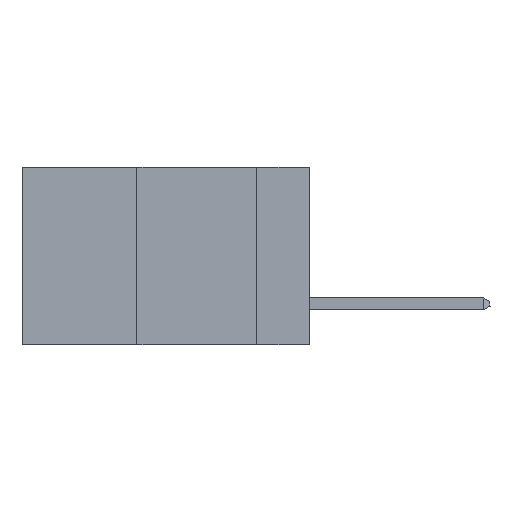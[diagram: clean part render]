
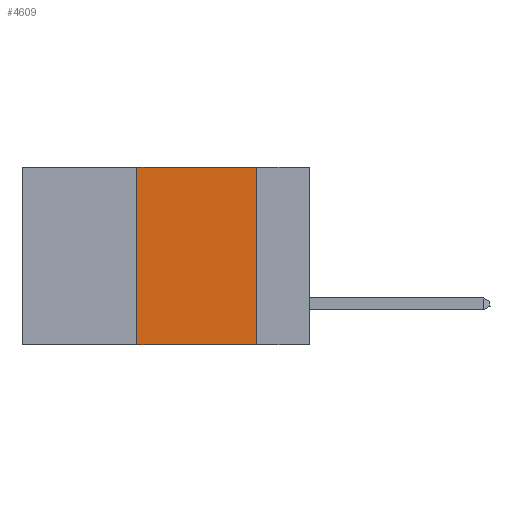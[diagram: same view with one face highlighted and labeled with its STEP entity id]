
A CAD part, left-side view. The second image highlights one B-rep face of the part: STEP entity #4609.
In plain terms, the highlighted planar face has unit normal (-1, 0, 0).
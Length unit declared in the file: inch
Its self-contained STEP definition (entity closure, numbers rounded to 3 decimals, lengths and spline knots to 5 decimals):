
#350 = VECTOR ( 'NONE', #17200, 39.37008 ) ;
#497 = VERTEX_POINT ( 'NONE', #6033 ) ;
#723 = AXIS2_PLACEMENT_3D ( 'NONE', #917, #4396, #20403 ) ;
#917 = CARTESIAN_POINT ( 'NONE',  ( 0., 0.6, 0. ) ) ;
#1806 = EDGE_CURVE ( 'NONE', #2650, #6221, #4624, .T. ) ;
#2217 = EDGE_CURVE ( 'NONE', #2650, #497, #7634, .T. ) ;
#2650 = VERTEX_POINT ( 'NONE', #16991 ) ;
#2866 = ORIENTED_EDGE ( 'NONE', *, *, #17367, .F. ) ;
#3147 = VERTEX_POINT ( 'NONE', #14581 ) ;
#3771 = VECTOR ( 'NONE', #6370, 39.37008 ) ;
#3840 = CARTESIAN_POINT ( 'NONE',  ( 0., 0.11, -0.37 ) ) ;
#4396 = DIRECTION ( 'NONE',  ( 1., 0., 0. ) ) ;
#4609 = ADVANCED_FACE ( 'NONE', ( #16020 ), #13310, .F. ) ;
#4624 = LINE ( 'NONE', #15113, #9568 ) ;
#5716 = EDGE_LOOP ( 'NONE', ( #9611, #2866, #8978, #10010 ) ) ;
#5736 = LINE ( 'NONE', #20801, #6278 ) ;
#6033 = CARTESIAN_POINT ( 'NONE',  ( 0., 0.36, 0. ) ) ;
#6221 = VERTEX_POINT ( 'NONE', #3840 ) ;
#6278 = VECTOR ( 'NONE', #22473, 39.37008 ) ;
#6370 = DIRECTION ( 'NONE',  ( 0., 0., 1. ) ) ;
#7634 = LINE ( 'NONE', #20424, #3771 ) ;
#8950 = LINE ( 'NONE', #22598, #350 ) ;
#8978 = ORIENTED_EDGE ( 'NONE', *, *, #2217, .F. ) ;
#9568 = VECTOR ( 'NONE', #18700, 39.37008 ) ;
#9611 = ORIENTED_EDGE ( 'NONE', *, *, #14842, .F. ) ;
#10010 = ORIENTED_EDGE ( 'NONE', *, *, #1806, .T. ) ;
#13310 = PLANE ( 'NONE',  #723 ) ;
#14581 = CARTESIAN_POINT ( 'NONE',  ( 0., 0.11, 0. ) ) ;
#14842 = EDGE_CURVE ( 'NONE', #3147, #6221, #5736, .T. ) ;
#15113 = CARTESIAN_POINT ( 'NONE',  ( 0., 0.6, -0.37 ) ) ;
#16020 = FACE_OUTER_BOUND ( 'NONE', #5716, .T. ) ;
#16991 = CARTESIAN_POINT ( 'NONE',  ( 0., 0.36, -0.37 ) ) ;
#17200 = DIRECTION ( 'NONE',  ( 0., -1., 0. ) ) ;
#17367 = EDGE_CURVE ( 'NONE', #497, #3147, #8950, .T. ) ;
#18700 = DIRECTION ( 'NONE',  ( 0., -1., 0. ) ) ;
#20403 = DIRECTION ( 'NONE',  ( 0., 0., -1. ) ) ;
#20424 = CARTESIAN_POINT ( 'NONE',  ( 0., 0.36, 0. ) ) ;
#20801 = CARTESIAN_POINT ( 'NONE',  ( 0., 0.11, 0. ) ) ;
#22473 = DIRECTION ( 'NONE',  ( 0., 0., -1. ) ) ;
#22598 = CARTESIAN_POINT ( 'NONE',  ( 0., 0.6, 0. ) ) ;
